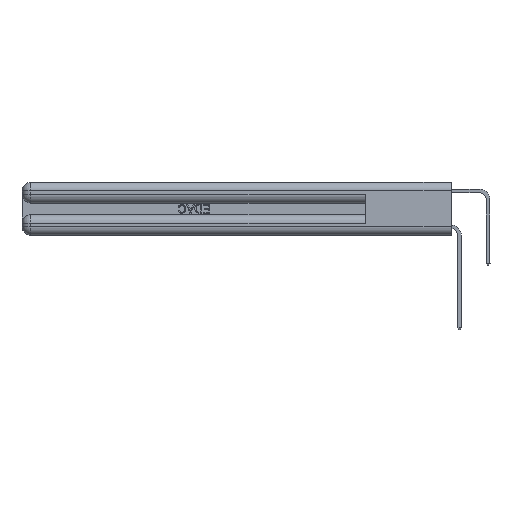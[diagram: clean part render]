
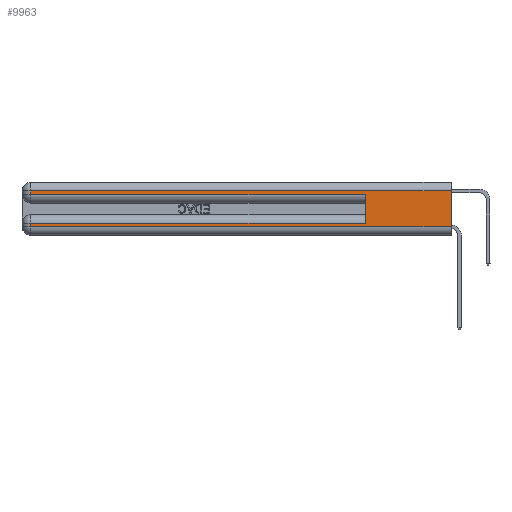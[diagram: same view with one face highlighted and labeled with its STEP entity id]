
A CAD part, left-side view. The second image highlights one B-rep face of the part: STEP entity #9963.
In plain terms, the highlighted planar face has unit normal (-1, 0, 0).
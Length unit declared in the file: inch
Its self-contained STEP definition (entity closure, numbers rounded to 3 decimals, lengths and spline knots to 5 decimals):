
#348 = CARTESIAN_POINT ( 'NONE',  ( 0., 0., 0.285 ) ) ;
#363 = LINE ( 'NONE', #16417, #4762 ) ;
#451 = CARTESIAN_POINT ( 'NONE',  ( 0., 2.94, 0.37 ) ) ;
#863 = LINE ( 'NONE', #19586, #14082 ) ;
#1058 = DIRECTION ( 'NONE',  ( 0., -1., 0. ) ) ;
#1087 = LINE ( 'NONE', #348, #2969 ) ;
#2465 = CARTESIAN_POINT ( 'NONE',  ( 0., 0.6, 0.085 ) ) ;
#2969 = VECTOR ( 'NONE', #1058, 39.37008 ) ;
#3081 = ORIENTED_EDGE ( 'NONE', *, *, #16001, .T. ) ;
#3352 = LINE ( 'NONE', #16406, #21294 ) ;
#4762 = VECTOR ( 'NONE', #21215, 39.37008 ) ;
#5071 = LINE ( 'NONE', #30037, #16079 ) ;
#5897 = ORIENTED_EDGE ( 'NONE', *, *, #21485, .T. ) ;
#5917 = PLANE ( 'NONE',  #13783 ) ;
#5984 = CARTESIAN_POINT ( 'NONE',  ( 0., 0., 0.31 ) ) ;
#7875 = DIRECTION ( 'NONE',  ( 0., 0., -1. ) ) ;
#7884 = FACE_OUTER_BOUND ( 'NONE', #24104, .T. ) ;
#8066 = DIRECTION ( 'NONE',  ( 1., 0., 0. ) ) ;
#8099 = VECTOR ( 'NONE', #22618, 39.37008 ) ;
#8259 = VERTEX_POINT ( 'NONE', #15508 ) ;
#8862 = CARTESIAN_POINT ( 'NONE',  ( 0., 2.94, 0.31 ) ) ;
#9963 = ADVANCED_FACE ( 'NONE', ( #7884 ), #5917, .F. ) ;
#10309 = VERTEX_POINT ( 'NONE', #8862 ) ;
#11067 = VERTEX_POINT ( 'NONE', #29538 ) ;
#11752 = LINE ( 'NONE', #27507, #22747 ) ;
#11886 = VERTEX_POINT ( 'NONE', #2465 ) ;
#12110 = DIRECTION ( 'NONE',  ( 0., 0., -1. ) ) ;
#12985 = VERTEX_POINT ( 'NONE', #13540 ) ;
#13540 = CARTESIAN_POINT ( 'NONE',  ( 0., 2.94, 0.285 ) ) ;
#13546 = VERTEX_POINT ( 'NONE', #22476 ) ;
#13783 = AXIS2_PLACEMENT_3D ( 'NONE', #21882, #8066, #7875 ) ;
#13837 = LINE ( 'NONE', #451, #19340 ) ;
#14082 = VECTOR ( 'NONE', #29126, 39.37008 ) ;
#14819 = EDGE_CURVE ( 'NONE', #11886, #13546, #16913, .T. ) ;
#15508 = CARTESIAN_POINT ( 'NONE',  ( 0., 0., 0.06 ) ) ;
#15547 = EDGE_CURVE ( 'NONE', #12985, #13546, #1087, .T. ) ;
#15565 = ORIENTED_EDGE ( 'NONE', *, *, #16455, .F. ) ;
#16001 = EDGE_CURVE ( 'NONE', #11067, #16468, #363, .T. ) ;
#16079 = VECTOR ( 'NONE', #25344, 39.37008 ) ;
#16406 = CARTESIAN_POINT ( 'NONE',  ( 0., 0., 0.06 ) ) ;
#16417 = CARTESIAN_POINT ( 'NONE',  ( 0., 2.94, 0.37 ) ) ;
#16455 = EDGE_CURVE ( 'NONE', #19090, #8259, #5071, .T. ) ;
#16468 = VERTEX_POINT ( 'NONE', #27876 ) ;
#16702 = DIRECTION ( 'NONE',  ( 0., -1., 0. ) ) ;
#16913 = LINE ( 'NONE', #22521, #8099 ) ;
#17159 = ORIENTED_EDGE ( 'NONE', *, *, #15547, .T. ) ;
#17276 = EDGE_CURVE ( 'NONE', #10309, #12985, #13837, .T. ) ;
#19090 = VERTEX_POINT ( 'NONE', #5984 ) ;
#19259 = ORIENTED_EDGE ( 'NONE', *, *, #21486, .T. ) ;
#19340 = VECTOR ( 'NONE', #12110, 39.37008 ) ;
#19586 = CARTESIAN_POINT ( 'NONE',  ( 0., 0., 0.085 ) ) ;
#19630 = EDGE_CURVE ( 'NONE', #11886, #11067, #863, .T. ) ;
#21013 = DIRECTION ( 'NONE',  ( 0., 1., 0. ) ) ;
#21215 = DIRECTION ( 'NONE',  ( 0., 0., -1. ) ) ;
#21294 = VECTOR ( 'NONE', #16702, 39.37008 ) ;
#21357 = ORIENTED_EDGE ( 'NONE', *, *, #17276, .T. ) ;
#21485 = EDGE_CURVE ( 'NONE', #19090, #10309, #11752, .T. ) ;
#21486 = EDGE_CURVE ( 'NONE', #16468, #8259, #3352, .T. ) ;
#21882 = CARTESIAN_POINT ( 'NONE',  ( 0., 0., 0.37 ) ) ;
#22476 = CARTESIAN_POINT ( 'NONE',  ( 0., 0.6, 0.285 ) ) ;
#22521 = CARTESIAN_POINT ( 'NONE',  ( 0., 0.6, 0.145 ) ) ;
#22618 = DIRECTION ( 'NONE',  ( 0., 0., 1. ) ) ;
#22747 = VECTOR ( 'NONE', #21013, 39.37008 ) ;
#24104 = EDGE_LOOP ( 'NONE', ( #15565, #5897, #21357, #17159, #26871, #25942, #3081, #19259 ) ) ;
#25344 = DIRECTION ( 'NONE',  ( 0., 0., -1. ) ) ;
#25942 = ORIENTED_EDGE ( 'NONE', *, *, #19630, .T. ) ;
#26871 = ORIENTED_EDGE ( 'NONE', *, *, #14819, .F. ) ;
#27507 = CARTESIAN_POINT ( 'NONE',  ( 0., 0., 0.31 ) ) ;
#27876 = CARTESIAN_POINT ( 'NONE',  ( 0., 2.94, 0.06 ) ) ;
#29126 = DIRECTION ( 'NONE',  ( 0., 1., 0. ) ) ;
#29538 = CARTESIAN_POINT ( 'NONE',  ( 0., 2.94, 0.085 ) ) ;
#30037 = CARTESIAN_POINT ( 'NONE',  ( 0., 0., 0.37 ) ) ;
